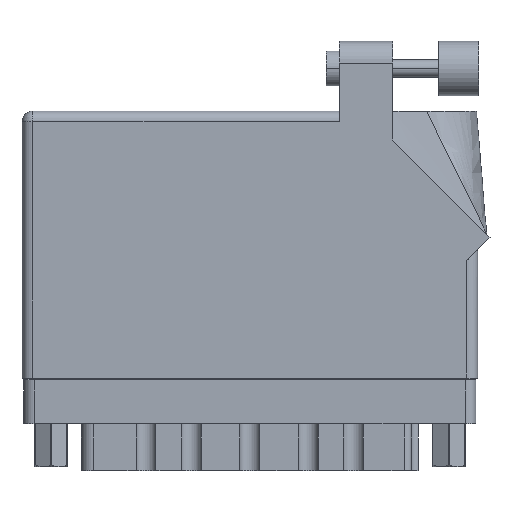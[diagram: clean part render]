
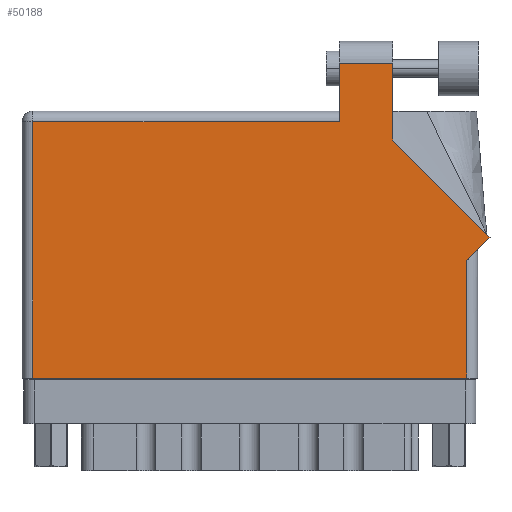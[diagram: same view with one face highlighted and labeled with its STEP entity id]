
A CAD part, front view. The second image highlights one B-rep face of the part: STEP entity #50188.
In plain terms, the highlighted face is planar.
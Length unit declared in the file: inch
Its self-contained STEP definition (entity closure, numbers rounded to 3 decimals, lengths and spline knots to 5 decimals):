
#452 = VERTEX_POINT ( 'NONE', #29565 ) ;
#2711 = CARTESIAN_POINT ( 'NONE',  ( 2.126, 1.805, 0. ) ) ;
#4851 = EDGE_CURVE ( 'NONE', #31942, #55813, #35306, .T. ) ;
#4977 = CARTESIAN_POINT ( 'NONE',  ( 0., 0., 0. ) ) ;
#5137 = VERTEX_POINT ( 'NONE', #39921 ) ;
#5223 = EDGE_CURVE ( 'NONE', #43062, #31942, #26191, .T. ) ;
#7293 = DIRECTION ( 'NONE',  ( 0., 1., 0. ) ) ;
#7632 = ORIENTED_EDGE ( 'NONE', *, *, #51304, .T. ) ;
#8130 = CARTESIAN_POINT ( 'NONE',  ( 2.126, 1.36442, 0. ) ) ;
#8425 = EDGE_CURVE ( 'NONE', #35970, #43062, #32391, .T. ) ;
#13323 = ORIENTED_EDGE ( 'NONE', *, *, #41172, .T. ) ;
#14632 = CARTESIAN_POINT ( 'NONE',  ( 1.819, 1.53, 0. ) ) ;
#14856 = DIRECTION ( 'NONE',  ( 0.707, 0.707, 0. ) ) ;
#15712 = AXIS2_PLACEMENT_3D ( 'NONE', #15815, #46669, #51187 ) ;
#15815 = CARTESIAN_POINT ( 'NONE',  ( 0., 1.53, 0. ) ) ;
#17630 = DIRECTION ( 'NONE',  ( 1., 0., 0. ) ) ;
#19836 = ORIENTED_EDGE ( 'NONE', *, *, #8425, .T. ) ;
#20668 = EDGE_CURVE ( 'NONE', #452, #35970, #33258, .T. ) ;
#20796 = CARTESIAN_POINT ( 'NONE',  ( 0., 1.468, 0. ) ) ;
#21141 = VERTEX_POINT ( 'NONE', #47891 ) ;
#21964 = EDGE_CURVE ( 'NONE', #55813, #21141, #52609, .T. ) ;
#22558 = VECTOR ( 'NONE', #27513, 39.37008 ) ;
#23096 = CARTESIAN_POINT ( 'NONE',  ( 2.612, 0.737, 0. ) ) ;
#24697 = CARTESIAN_POINT ( 'NONE',  ( 0.062, 1.468, 0. ) ) ;
#25949 = EDGE_LOOP ( 'NONE', ( #43010, #19836, #35518, #55935, #49517, #35402, #7632, #13323, #36393 ) ) ;
#26191 = LINE ( 'NONE', #14632, #43654 ) ;
#27164 = CARTESIAN_POINT ( 'NONE',  ( 2.55, 0., 0. ) ) ;
#27397 = LINE ( 'NONE', #56492, #31604 ) ;
#27513 = DIRECTION ( 'NONE',  ( 0., -1., 0. ) ) ;
#27655 = VECTOR ( 'NONE', #31166, 39.37008 ) ;
#29565 = CARTESIAN_POINT ( 'NONE',  ( 2.126, 1.36442, 0. ) ) ;
#31107 = EDGE_CURVE ( 'NONE', #5137, #452, #39441, .T. ) ;
#31166 = DIRECTION ( 'NONE',  ( 0., 1., 0. ) ) ;
#31604 = VECTOR ( 'NONE', #7293, 39.37008 ) ;
#31942 = VERTEX_POINT ( 'NONE', #42616 ) ;
#32017 = CARTESIAN_POINT ( 'NONE',  ( 0.062, 0., 0. ) ) ;
#32391 = LINE ( 'NONE', #39775, #32985 ) ;
#32985 = VECTOR ( 'NONE', #53053, 39.37008 ) ;
#33258 = LINE ( 'NONE', #8130, #27655 ) ;
#33568 = CARTESIAN_POINT ( 'NONE',  ( 1.819, 1.805, 0. ) ) ;
#34469 = DIRECTION ( 'NONE',  ( -1., 0., 0. ) ) ;
#35306 = LINE ( 'NONE', #20796, #46442 ) ;
#35402 = ORIENTED_EDGE ( 'NONE', *, *, #43235, .T. ) ;
#35518 = ORIENTED_EDGE ( 'NONE', *, *, #5223, .T. ) ;
#35970 = VERTEX_POINT ( 'NONE', #2711 ) ;
#36321 = DIRECTION ( 'NONE',  ( 0., -1., 0. ) ) ;
#36393 = ORIENTED_EDGE ( 'NONE', *, *, #31107, .T. ) ;
#36793 = CARTESIAN_POINT ( 'NONE',  ( 2.55, 0.675, 0. ) ) ;
#39441 = LINE ( 'NONE', #41174, #45031 ) ;
#39775 = CARTESIAN_POINT ( 'NONE',  ( 1.819, 1.805, 0. ) ) ;
#39921 = CARTESIAN_POINT ( 'NONE',  ( 2.68271, 0.80771, 0. ) ) ;
#40803 = DIRECTION ( 'NONE',  ( -0.707, 0.707, 0. ) ) ;
#41172 = EDGE_CURVE ( 'NONE', #52239, #5137, #54980, .T. ) ;
#41174 = CARTESIAN_POINT ( 'NONE',  ( 2.68271, 0.80771, 0. ) ) ;
#41723 = VECTOR ( 'NONE', #14856, 39.37008 ) ;
#42196 = PLANE ( 'NONE',  #15712 ) ;
#42616 = CARTESIAN_POINT ( 'NONE',  ( 1.819, 1.468, 0. ) ) ;
#42868 = FACE_OUTER_BOUND ( 'NONE', #25949, .T. ) ;
#43010 = ORIENTED_EDGE ( 'NONE', *, *, #20668, .T. ) ;
#43062 = VERTEX_POINT ( 'NONE', #33568 ) ;
#43235 = EDGE_CURVE ( 'NONE', #21141, #56177, #44017, .T. ) ;
#43654 = VECTOR ( 'NONE', #36321, 39.37008 ) ;
#44017 = LINE ( 'NONE', #4977, #48222 ) ;
#45031 = VECTOR ( 'NONE', #40803, 39.37008 ) ;
#46442 = VECTOR ( 'NONE', #34469, 39.37008 ) ;
#46669 = DIRECTION ( 'NONE',  ( 0., 0., -1. ) ) ;
#47891 = CARTESIAN_POINT ( 'NONE',  ( 0.062, 0., 0. ) ) ;
#48222 = VECTOR ( 'NONE', #17630, 39.37008 ) ;
#49517 = ORIENTED_EDGE ( 'NONE', *, *, #21964, .T. ) ;
#50188 = ADVANCED_FACE ( 'NONE', ( #42868 ), #42196, .F. ) ;
#51187 = DIRECTION ( 'NONE',  ( -1., 0., 0. ) ) ;
#51304 = EDGE_CURVE ( 'NONE', #56177, #52239, #27397, .T. ) ;
#52239 = VERTEX_POINT ( 'NONE', #36793 ) ;
#52609 = LINE ( 'NONE', #32017, #22558 ) ;
#53053 = DIRECTION ( 'NONE',  ( -1., 0., 0. ) ) ;
#54980 = LINE ( 'NONE', #23096, #41723 ) ;
#55813 = VERTEX_POINT ( 'NONE', #24697 ) ;
#55935 = ORIENTED_EDGE ( 'NONE', *, *, #4851, .T. ) ;
#56177 = VERTEX_POINT ( 'NONE', #27164 ) ;
#56492 = CARTESIAN_POINT ( 'NONE',  ( 2.55, 0.737, 0. ) ) ;
